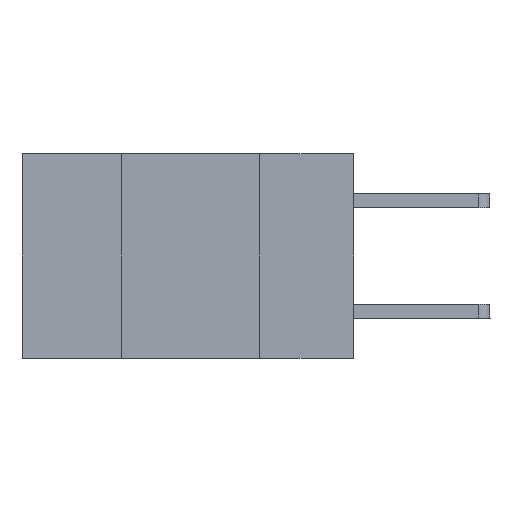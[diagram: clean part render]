
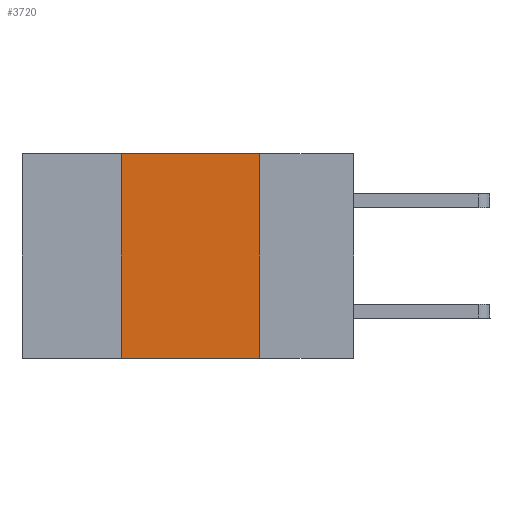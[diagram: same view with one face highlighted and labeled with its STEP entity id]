
A CAD part, left-side view. The second image highlights one B-rep face of the part: STEP entity #3720.
In plain terms, the highlighted planar face has unit normal (-1, 0, 0).
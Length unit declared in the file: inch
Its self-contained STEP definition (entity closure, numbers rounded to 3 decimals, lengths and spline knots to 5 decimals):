
#150 = LINE ( 'NONE', #12629, #7115 ) ;
#468 = CARTESIAN_POINT ( 'NONE',  ( 0., 0.17, 0. ) ) ;
#494 = EDGE_LOOP ( 'NONE', ( #12829, #10022, #3520, #8741 ) ) ;
#1687 = AXIS2_PLACEMENT_3D ( 'NONE', #7386, #6245, #3987 ) ;
#2323 = DIRECTION ( 'NONE',  ( 0., -1., 0. ) ) ;
#2772 = FACE_OUTER_BOUND ( 'NONE', #494, .T. ) ;
#3211 = EDGE_CURVE ( 'NONE', #11417, #14220, #5988, .T. ) ;
#3401 = CARTESIAN_POINT ( 'NONE',  ( 0., 0.42, 0. ) ) ;
#3520 = ORIENTED_EDGE ( 'NONE', *, *, #3211, .F. ) ;
#3720 = ADVANCED_FACE ( 'NONE', ( #2772 ), #4219, .F. ) ;
#3987 = DIRECTION ( 'NONE',  ( 0., 0., -1. ) ) ;
#4038 = EDGE_CURVE ( 'NONE', #11417, #8208, #12348, .T. ) ;
#4219 = PLANE ( 'NONE',  #1687 ) ;
#5053 = DIRECTION ( 'NONE',  ( 0., 0., -1. ) ) ;
#5352 = VERTEX_POINT ( 'NONE', #10192 ) ;
#5988 = LINE ( 'NONE', #7339, #6475 ) ;
#6125 = VECTOR ( 'NONE', #5053, 39.37008 ) ;
#6245 = DIRECTION ( 'NONE',  ( 1., 0., 0. ) ) ;
#6280 = DIRECTION ( 'NONE',  ( 0., 0., 1. ) ) ;
#6409 = LINE ( 'NONE', #468, #6125 ) ;
#6475 = VECTOR ( 'NONE', #6280, 39.37008 ) ;
#6717 = CARTESIAN_POINT ( 'NONE',  ( 0., 0.42, -0.37 ) ) ;
#7115 = VECTOR ( 'NONE', #2323, 39.37008 ) ;
#7242 = CARTESIAN_POINT ( 'NONE',  ( 0., 0.17, -0.37 ) ) ;
#7339 = CARTESIAN_POINT ( 'NONE',  ( 0., 0.42, 0. ) ) ;
#7386 = CARTESIAN_POINT ( 'NONE',  ( 0., 0.6, 0. ) ) ;
#8208 = VERTEX_POINT ( 'NONE', #7242 ) ;
#8496 = EDGE_CURVE ( 'NONE', #5352, #8208, #6409, .T. ) ;
#8741 = ORIENTED_EDGE ( 'NONE', *, *, #4038, .T. ) ;
#9040 = CARTESIAN_POINT ( 'NONE',  ( 0., 0.6, -0.37 ) ) ;
#9864 = VECTOR ( 'NONE', #13541, 39.37008 ) ;
#10022 = ORIENTED_EDGE ( 'NONE', *, *, #13219, .F. ) ;
#10192 = CARTESIAN_POINT ( 'NONE',  ( 0., 0.17, 0. ) ) ;
#11417 = VERTEX_POINT ( 'NONE', #6717 ) ;
#12348 = LINE ( 'NONE', #9040, #9864 ) ;
#12629 = CARTESIAN_POINT ( 'NONE',  ( 0., 0.6, 0. ) ) ;
#12829 = ORIENTED_EDGE ( 'NONE', *, *, #8496, .F. ) ;
#13219 = EDGE_CURVE ( 'NONE', #14220, #5352, #150, .T. ) ;
#13541 = DIRECTION ( 'NONE',  ( 0., -1., 0. ) ) ;
#14220 = VERTEX_POINT ( 'NONE', #3401 ) ;
